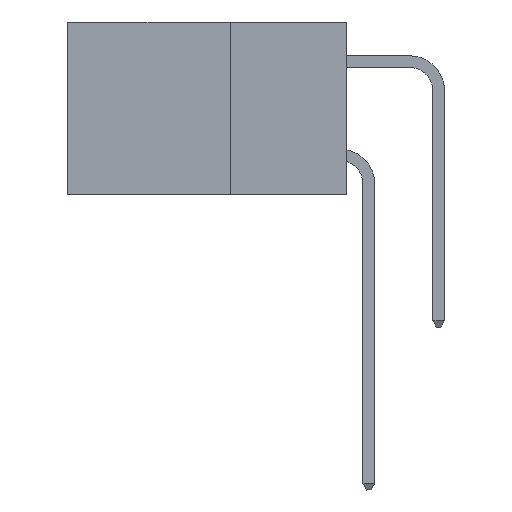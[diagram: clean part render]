
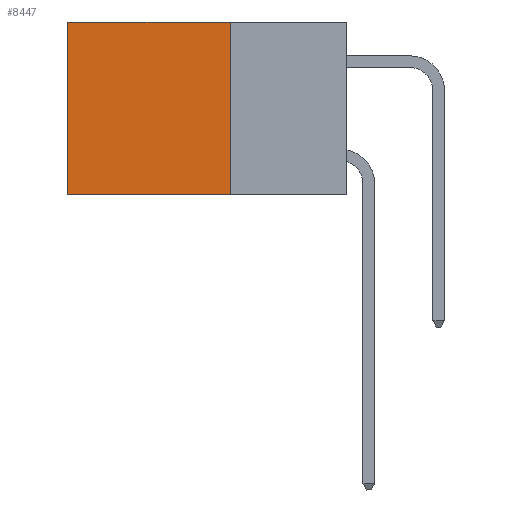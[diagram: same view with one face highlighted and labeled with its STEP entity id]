
A CAD part, left-side view. The second image highlights one B-rep face of the part: STEP entity #8447.
In plain terms, the highlighted planar face has unit normal (-1, 0, 0).
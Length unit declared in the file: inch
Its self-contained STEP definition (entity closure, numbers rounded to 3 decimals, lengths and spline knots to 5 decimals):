
#141 = LINE ( 'NONE', #12692, #6742 ) ;
#526 = ORIENTED_EDGE ( 'NONE', *, *, #10920, .T. ) ;
#586 = LINE ( 'NONE', #1424, #10832 ) ;
#1215 = CARTESIAN_POINT ( 'NONE',  ( 0.2875, 0.6, 0. ) ) ;
#1424 = CARTESIAN_POINT ( 'NONE',  ( 0.2875, 0.25, 0. ) ) ;
#1827 = DIRECTION ( 'NONE',  ( 0., 0., -1. ) ) ;
#2390 = EDGE_CURVE ( 'NONE', #8944, #13420, #2859, .T. ) ;
#2859 = LINE ( 'NONE', #16236, #15794 ) ;
#3353 = PLANE ( 'NONE',  #6452 ) ;
#4013 = DIRECTION ( 'NONE',  ( 0., 0., -1. ) ) ;
#5371 = CARTESIAN_POINT ( 'NONE',  ( 0.2875, 0.25, 0. ) ) ;
#6244 = ORIENTED_EDGE ( 'NONE', *, *, #6345, .F. ) ;
#6345 = EDGE_CURVE ( 'NONE', #11324, #8944, #141, .T. ) ;
#6452 = AXIS2_PLACEMENT_3D ( 'NONE', #13336, #15842, #8398 ) ;
#6742 = VECTOR ( 'NONE', #4013, 39.37008 ) ;
#6926 = DIRECTION ( 'NONE',  ( 0., 1., 0. ) ) ;
#6965 = CARTESIAN_POINT ( 'NONE',  ( 0.2875, 0.6, 0. ) ) ;
#7800 = FACE_OUTER_BOUND ( 'NONE', #9665, .T. ) ;
#8398 = DIRECTION ( 'NONE',  ( 0., 0., -1. ) ) ;
#8447 = ADVANCED_FACE ( 'NONE', ( #7800 ), #3353, .F. ) ;
#8773 = ORIENTED_EDGE ( 'NONE', *, *, #11984, .T. ) ;
#8944 = VERTEX_POINT ( 'NONE', #12921 ) ;
#9333 = ORIENTED_EDGE ( 'NONE', *, *, #2390, .F. ) ;
#9553 = CARTESIAN_POINT ( 'NONE',  ( 0.2875, 0.6, -0.37 ) ) ;
#9665 = EDGE_LOOP ( 'NONE', ( #526, #9333, #6244, #8773 ) ) ;
#10078 = VECTOR ( 'NONE', #1827, 39.37008 ) ;
#10384 = DIRECTION ( 'NONE',  ( 0., 1., 0. ) ) ;
#10832 = VECTOR ( 'NONE', #10384, 39.37008 ) ;
#10920 = EDGE_CURVE ( 'NONE', #15249, #13420, #13342, .T. ) ;
#11324 = VERTEX_POINT ( 'NONE', #5371 ) ;
#11984 = EDGE_CURVE ( 'NONE', #11324, #15249, #586, .T. ) ;
#12692 = CARTESIAN_POINT ( 'NONE',  ( 0.2875, 0.25, 0. ) ) ;
#12921 = CARTESIAN_POINT ( 'NONE',  ( 0.2875, 0.25, -0.37 ) ) ;
#13336 = CARTESIAN_POINT ( 'NONE',  ( 0.2875, 0.25, 0. ) ) ;
#13342 = LINE ( 'NONE', #6965, #10078 ) ;
#13420 = VERTEX_POINT ( 'NONE', #9553 ) ;
#15249 = VERTEX_POINT ( 'NONE', #1215 ) ;
#15794 = VECTOR ( 'NONE', #6926, 39.37008 ) ;
#15842 = DIRECTION ( 'NONE',  ( 1., 0., 0. ) ) ;
#16236 = CARTESIAN_POINT ( 'NONE',  ( 0.2875, 0.25, -0.37 ) ) ;
